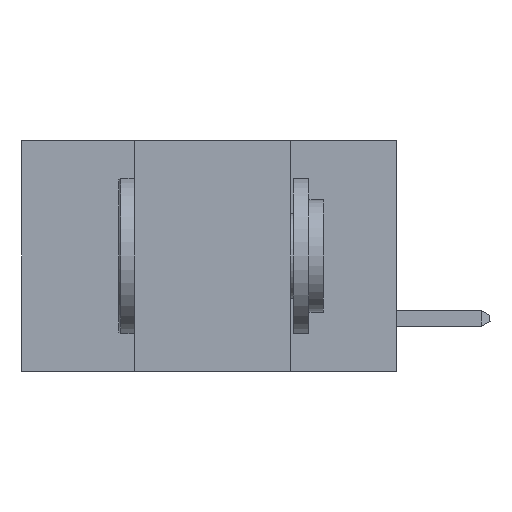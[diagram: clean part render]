
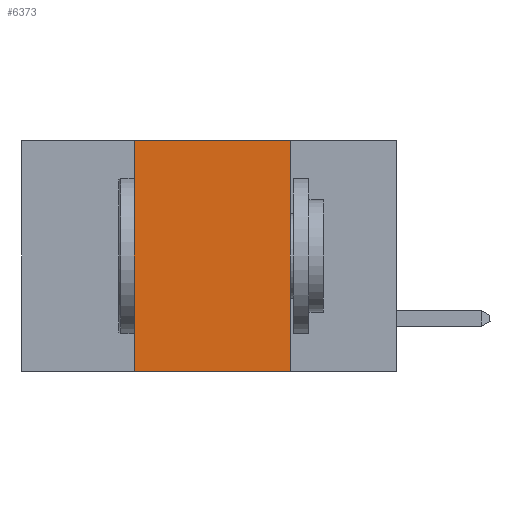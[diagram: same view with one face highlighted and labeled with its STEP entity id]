
A CAD part, left-side view. The second image highlights one B-rep face of the part: STEP entity #6373.
In plain terms, the highlighted planar face has unit normal (-1, 0, 0).
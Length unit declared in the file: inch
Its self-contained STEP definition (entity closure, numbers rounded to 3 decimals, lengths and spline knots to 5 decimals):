
#967 = VERTEX_POINT ( 'NONE', #18074 ) ;
#2861 = CARTESIAN_POINT ( 'NONE',  ( 0., 0.17, 0. ) ) ;
#3030 = EDGE_CURVE ( 'NONE', #26523, #3457, #14377, .T. ) ;
#3457 = VERTEX_POINT ( 'NONE', #16272 ) ;
#4310 = FACE_OUTER_BOUND ( 'NONE', #14888, .T. ) ;
#5658 = CARTESIAN_POINT ( 'NONE',  ( 0., 0.42, 0. ) ) ;
#6373 = ADVANCED_FACE ( 'NONE', ( #4310 ), #19357, .F. ) ;
#7270 = DIRECTION ( 'NONE',  ( 0., -1., 0. ) ) ;
#7957 = DIRECTION ( 'NONE',  ( 0., 0., 1. ) ) ;
#8261 = DIRECTION ( 'NONE',  ( 0., 0., -1. ) ) ;
#8378 = EDGE_CURVE ( 'NONE', #967, #21353, #9413, .T. ) ;
#9179 = CARTESIAN_POINT ( 'NONE',  ( 0., 0.42, 0. ) ) ;
#9413 = LINE ( 'NONE', #24083, #20513 ) ;
#12697 = CARTESIAN_POINT ( 'NONE',  ( 0., 0.6, 0. ) ) ;
#13182 = ORIENTED_EDGE ( 'NONE', *, *, #15862, .F. ) ;
#14377 = LINE ( 'NONE', #14530, #26126 ) ;
#14530 = CARTESIAN_POINT ( 'NONE',  ( 0., 0.6, 0. ) ) ;
#14667 = LINE ( 'NONE', #2861, #19181 ) ;
#14888 = EDGE_LOOP ( 'NONE', ( #27984, #17682, #13182, #24970 ) ) ;
#15252 = LINE ( 'NONE', #5658, #26296 ) ;
#15862 = EDGE_CURVE ( 'NONE', #967, #26523, #15252, .T. ) ;
#16272 = CARTESIAN_POINT ( 'NONE',  ( 0., 0.17, 0. ) ) ;
#17682 = ORIENTED_EDGE ( 'NONE', *, *, #3030, .F. ) ;
#18074 = CARTESIAN_POINT ( 'NONE',  ( 0., 0.42, -0.37 ) ) ;
#19181 = VECTOR ( 'NONE', #27405, 39.37008 ) ;
#19188 = CARTESIAN_POINT ( 'NONE',  ( 0., 0.17, -0.37 ) ) ;
#19357 = PLANE ( 'NONE',  #28532 ) ;
#20513 = VECTOR ( 'NONE', #26255, 39.37008 ) ;
#21353 = VERTEX_POINT ( 'NONE', #19188 ) ;
#21585 = DIRECTION ( 'NONE',  ( 1., 0., 0. ) ) ;
#21800 = EDGE_CURVE ( 'NONE', #3457, #21353, #14667, .T. ) ;
#24083 = CARTESIAN_POINT ( 'NONE',  ( 0., 0.6, -0.37 ) ) ;
#24970 = ORIENTED_EDGE ( 'NONE', *, *, #8378, .T. ) ;
#26126 = VECTOR ( 'NONE', #7270, 39.37008 ) ;
#26255 = DIRECTION ( 'NONE',  ( 0., -1., 0. ) ) ;
#26296 = VECTOR ( 'NONE', #7957, 39.37008 ) ;
#26523 = VERTEX_POINT ( 'NONE', #9179 ) ;
#27405 = DIRECTION ( 'NONE',  ( 0., 0., -1. ) ) ;
#27984 = ORIENTED_EDGE ( 'NONE', *, *, #21800, .F. ) ;
#28532 = AXIS2_PLACEMENT_3D ( 'NONE', #12697, #21585, #8261 ) ;
